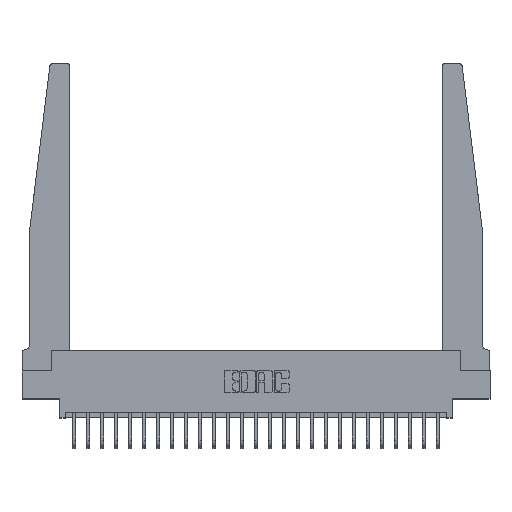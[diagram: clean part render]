
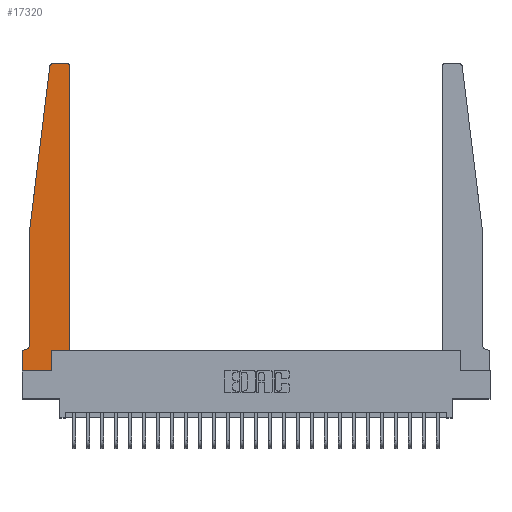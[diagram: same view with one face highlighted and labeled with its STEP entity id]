
A CAD part, top view. The second image highlights one B-rep face of the part: STEP entity #17320.
In plain terms, the highlighted planar face has unit normal (0, 0, 1).
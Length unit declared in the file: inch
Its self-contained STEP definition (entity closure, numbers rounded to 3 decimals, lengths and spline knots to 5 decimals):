
#844 = CARTESIAN_POINT ( 'NONE',  ( 0.065, 1.25, 0.37 ) ) ;
#1116 = ORIENTED_EDGE ( 'NONE', *, *, #19683, .T. ) ;
#1134 = VECTOR ( 'NONE', #7714, 39.37008 ) ;
#1173 = LINE ( 'NONE', #7192, #10469 ) ;
#1346 = VERTEX_POINT ( 'NONE', #21115 ) ;
#1653 = ORIENTED_EDGE ( 'NONE', *, *, #10418, .T. ) ;
#1702 = ORIENTED_EDGE ( 'NONE', *, *, #5513, .T. ) ;
#2764 = CIRCLE ( 'NONE', #20312, 0.05 ) ;
#2833 = DIRECTION ( 'NONE',  ( 0., -1., 0. ) ) ;
#3179 = ORIENTED_EDGE ( 'NONE', *, *, #23775, .T. ) ;
#3690 = CARTESIAN_POINT ( 'NONE',  ( 0.2605, 0.18, 0.37 ) ) ;
#4438 = CARTESIAN_POINT ( 'NONE',  ( 0.395, 2.72, 0.37 ) ) ;
#4597 = EDGE_CURVE ( 'NONE', #10856, #17145, #18415, .T. ) ;
#4611 = CARTESIAN_POINT ( 'NONE',  ( 0.065, 1.25, 0.37 ) ) ;
#4671 = VERTEX_POINT ( 'NONE', #14106 ) ;
#4807 = VERTEX_POINT ( 'NONE', #19876 ) ;
#5003 = EDGE_CURVE ( 'NONE', #13559, #17888, #11580, .T. ) ;
#5209 = CARTESIAN_POINT ( 'NONE',  ( 0.015, 0.2375, 0.37 ) ) ;
#5456 = CARTESIAN_POINT ( 'NONE',  ( 0.2605, 0., 0.37 ) ) ;
#5513 = EDGE_CURVE ( 'NONE', #17888, #1346, #11531, .T. ) ;
#5540 = ORIENTED_EDGE ( 'NONE', *, *, #9867, .T. ) ;
#6330 = DIRECTION ( 'NONE',  ( 1., 0., 0. ) ) ;
#6672 = CARTESIAN_POINT ( 'NONE',  ( 0., 0., 0.37 ) ) ;
#6981 = ORIENTED_EDGE ( 'NONE', *, *, #4597, .T. ) ;
#7088 = DIRECTION ( 'NONE',  ( -1., 0., 0. ) ) ;
#7140 = VECTOR ( 'NONE', #16510, 39.37008 ) ;
#7192 = CARTESIAN_POINT ( 'NONE',  ( 0.425, 0.18, 0.37 ) ) ;
#7231 = ORIENTED_EDGE ( 'NONE', *, *, #18362, .T. ) ;
#7366 = EDGE_CURVE ( 'NONE', #10528, #10856, #12331, .T. ) ;
#7516 = CARTESIAN_POINT ( 'NONE',  ( 0.27653, 2.72, 0.37 ) ) ;
#7714 = DIRECTION ( 'NONE',  ( -1., 0., 0. ) ) ;
#8035 = VECTOR ( 'NONE', #21954, 39.37008 ) ;
#8079 = VERTEX_POINT ( 'NONE', #20818 ) ;
#8378 = ORIENTED_EDGE ( 'NONE', *, *, #20021, .T. ) ;
#8528 = DIRECTION ( 'NONE',  ( 1., 0., 0. ) ) ;
#9010 = AXIS2_PLACEMENT_3D ( 'NONE', #7516, #20246, #9359 ) ;
#9028 = DIRECTION ( 'NONE',  ( 0., 1., 0. ) ) ;
#9359 = DIRECTION ( 'NONE',  ( 1., 0., 0. ) ) ;
#9416 = CARTESIAN_POINT ( 'NONE',  ( 0.395, 2.75, 0.37 ) ) ;
#9616 = CARTESIAN_POINT ( 'NONE',  ( 0., 0.1875, 0.37 ) ) ;
#9699 = PLANE ( 'NONE',  #15389 ) ;
#9867 = EDGE_CURVE ( 'NONE', #19653, #4807, #13642, .T. ) ;
#10418 = EDGE_CURVE ( 'NONE', #18377, #13559, #10766, .T. ) ;
#10469 = VECTOR ( 'NONE', #9028, 39.37008 ) ;
#10528 = VERTEX_POINT ( 'NONE', #15664 ) ;
#10766 = CIRCLE ( 'NONE', #17302, 0.03 ) ;
#10856 = VERTEX_POINT ( 'NONE', #18348 ) ;
#11531 = CIRCLE ( 'NONE', #9010, 0.03 ) ;
#11540 = DIRECTION ( 'NONE',  ( 1., 0., 0. ) ) ;
#11580 = LINE ( 'NONE', #18610, #1134 ) ;
#12331 = LINE ( 'NONE', #20219, #8035 ) ;
#12629 = DIRECTION ( 'NONE',  ( -1., 0., 0. ) ) ;
#12701 = LINE ( 'NONE', #4611, #22340 ) ;
#12995 = EDGE_LOOP ( 'NONE', ( #14100, #1702, #1116, #5540, #18944, #3179, #16682, #6981, #20356, #8378, #7231, #1653 ) ) ;
#13085 = VECTOR ( 'NONE', #2833, 39.37008 ) ;
#13114 = FACE_OUTER_BOUND ( 'NONE', #12995, .T. ) ;
#13559 = VERTEX_POINT ( 'NONE', #9416 ) ;
#13600 = VECTOR ( 'NONE', #8528, 39.37008 ) ;
#13642 = LINE ( 'NONE', #844, #13085 ) ;
#14100 = ORIENTED_EDGE ( 'NONE', *, *, #5003, .T. ) ;
#14106 = CARTESIAN_POINT ( 'NONE',  ( 0.425, 0.18, 0.37 ) ) ;
#14721 = CARTESIAN_POINT ( 'NONE',  ( 0.425, 0.18, 0.37 ) ) ;
#15032 = CARTESIAN_POINT ( 'NONE',  ( 0.27653, 2.75, 0.37 ) ) ;
#15273 = VECTOR ( 'NONE', #21990, 39.37008 ) ;
#15369 = VECTOR ( 'NONE', #12629, 39.37008 ) ;
#15389 = AXIS2_PLACEMENT_3D ( 'NONE', #9616, #22400, #11540 ) ;
#15500 = VERTEX_POINT ( 'NONE', #22480 ) ;
#15664 = CARTESIAN_POINT ( 'NONE',  ( 0., 0.1875, 0.37 ) ) ;
#15935 = LINE ( 'NONE', #16275, #15369 ) ;
#16275 = CARTESIAN_POINT ( 'NONE',  ( 0.065, 0.1875, 0.37 ) ) ;
#16508 = EDGE_CURVE ( 'NONE', #17145, #8079, #21059, .T. ) ;
#16510 = DIRECTION ( 'NONE',  ( 0., 1., 0. ) ) ;
#16682 = ORIENTED_EDGE ( 'NONE', *, *, #7366, .T. ) ;
#17145 = VERTEX_POINT ( 'NONE', #5456 ) ;
#17251 = DIRECTION ( 'NONE',  ( 0., 0., 1. ) ) ;
#17266 = CARTESIAN_POINT ( 'NONE',  ( 0.065, 1.25, 0.37 ) ) ;
#17302 = AXIS2_PLACEMENT_3D ( 'NONE', #4438, #17251, #6330 ) ;
#17320 = ADVANCED_FACE ( 'NONE', ( #13114 ), #9699, .T. ) ;
#17888 = VERTEX_POINT ( 'NONE', #15032 ) ;
#17996 = DIRECTION ( 'NONE',  ( 0., 0., -1. ) ) ;
#18348 = CARTESIAN_POINT ( 'NONE',  ( 0., 0., 0.37 ) ) ;
#18362 = EDGE_CURVE ( 'NONE', #4671, #18377, #1173, .T. ) ;
#18377 = VERTEX_POINT ( 'NONE', #18426 ) ;
#18415 = LINE ( 'NONE', #6672, #13600 ) ;
#18426 = CARTESIAN_POINT ( 'NONE',  ( 0.425, 2.72, 0.37 ) ) ;
#18610 = CARTESIAN_POINT ( 'NONE',  ( 0.25, 2.75, 0.37 ) ) ;
#18944 = ORIENTED_EDGE ( 'NONE', *, *, #22588, .T. ) ;
#19653 = VERTEX_POINT ( 'NONE', #17266 ) ;
#19683 = EDGE_CURVE ( 'NONE', #1346, #19653, #12701, .T. ) ;
#19876 = CARTESIAN_POINT ( 'NONE',  ( 0.065, 0.2375, 0.37 ) ) ;
#20021 = EDGE_CURVE ( 'NONE', #8079, #4671, #20082, .T. ) ;
#20082 = LINE ( 'NONE', #14721, #15273 ) ;
#20219 = CARTESIAN_POINT ( 'NONE',  ( 0., 0., 0.37 ) ) ;
#20246 = DIRECTION ( 'NONE',  ( 0., 0., 1. ) ) ;
#20312 = AXIS2_PLACEMENT_3D ( 'NONE', #5209, #17996, #7088 ) ;
#20356 = ORIENTED_EDGE ( 'NONE', *, *, #16508, .T. ) ;
#20818 = CARTESIAN_POINT ( 'NONE',  ( 0.2605, 0.18, 0.37 ) ) ;
#21059 = LINE ( 'NONE', #3690, #7140 ) ;
#21115 = CARTESIAN_POINT ( 'NONE',  ( 0.24675, 2.72367, 0.37 ) ) ;
#21954 = DIRECTION ( 'NONE',  ( 0., -1., 0. ) ) ;
#21990 = DIRECTION ( 'NONE',  ( 1., 0., 0. ) ) ;
#22340 = VECTOR ( 'NONE', #22798, 39.37008 ) ;
#22400 = DIRECTION ( 'NONE',  ( 0., 0., 1. ) ) ;
#22480 = CARTESIAN_POINT ( 'NONE',  ( 0.015, 0.1875, 0.37 ) ) ;
#22588 = EDGE_CURVE ( 'NONE', #4807, #15500, #2764, .T. ) ;
#22798 = DIRECTION ( 'NONE',  ( -0.122, -0.992, 0. ) ) ;
#23775 = EDGE_CURVE ( 'NONE', #15500, #10528, #15935, .T. ) ;
